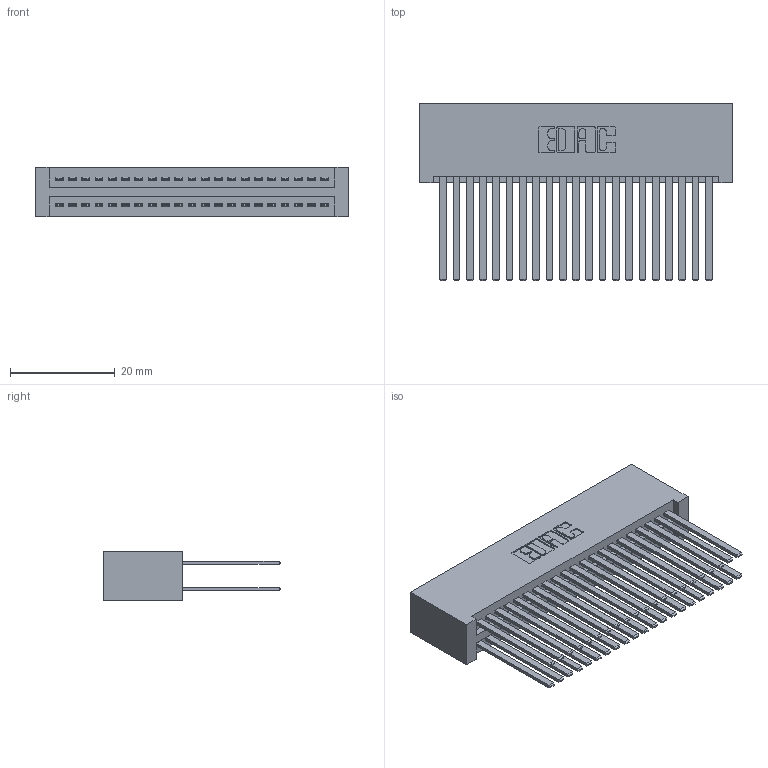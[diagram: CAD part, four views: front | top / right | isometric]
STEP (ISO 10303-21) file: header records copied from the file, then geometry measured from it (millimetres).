
FILE_DESCRIPTION (( 'STEP AP203' ), '1' );
FILE_NAME ('395-042-544-201.STEP', '2018-11-15T11:18:21', ( '' ), ( '' ), 'SwSTEP 2.0', 'SolidWorks 2016', '' );
FILE_SCHEMA (( 'CONFIG_CONTROL_DESIGN' ));
Length unit declared in the file: inch
Products named in the file (3): 345-292-001_345-293-144; 345 Part_No Mounting Lugs; 395-042-544-201
Assembly tree (43 placements, depth 2):
  395-042-544-201
    345 Part_No Mounting Lugs
    345-292-001_345-293-144  x42
Bounding box: 59.94 x 33.96 x 9.4 mm (x, y, z)
Volume: 6832.8 mm3; surface area: 11722.1 mm2
Topology: 43 solids, 43 shells, 1966 faces, 5819 edges, 3822 vertices
Faces by surface type: plane 1294, cylinder 672
Entity records: 18843 total; most frequent: CARTESIAN_POINT 3176, ORIENTED_EDGE 3110, DIRECTION 2819, EDGE_CURVE 1555, LINE 1351, VECTOR 1351, VERTEX_POINT 1034, AXIS2_PLACEMENT_3D 734
